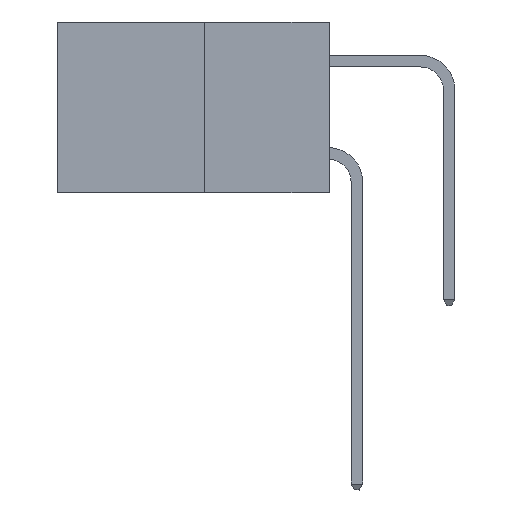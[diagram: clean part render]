
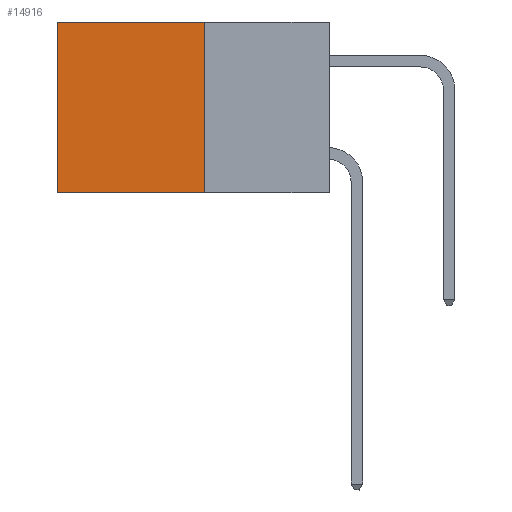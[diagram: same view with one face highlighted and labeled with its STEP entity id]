
A CAD part, left-side view. The second image highlights one B-rep face of the part: STEP entity #14916.
In plain terms, the highlighted planar face has unit normal (-1, 0, 0).
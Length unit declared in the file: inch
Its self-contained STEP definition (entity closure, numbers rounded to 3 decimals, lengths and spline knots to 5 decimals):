
#138 = EDGE_CURVE ( 'NONE', #4573, #4980, #4370, .T. ) ;
#1723 = EDGE_LOOP ( 'NONE', ( #2293, #3855, #4674, #15169 ) ) ;
#1887 = VECTOR ( 'NONE', #6535, 39.37008 ) ;
#2293 = ORIENTED_EDGE ( 'NONE', *, *, #6640, .T. ) ;
#2688 = PLANE ( 'NONE',  #4032 ) ;
#2776 = CARTESIAN_POINT ( 'NONE',  ( 0.277, 0.59, -0.37 ) ) ;
#3490 = EDGE_CURVE ( 'NONE', #12372, #6653, #14640, .T. ) ;
#3855 = ORIENTED_EDGE ( 'NONE', *, *, #138, .F. ) ;
#3945 = DIRECTION ( 'NONE',  ( 1., 0., 0. ) ) ;
#4032 = AXIS2_PLACEMENT_3D ( 'NONE', #12279, #3945, #12329 ) ;
#4370 = LINE ( 'NONE', #10048, #10388 ) ;
#4573 = VERTEX_POINT ( 'NONE', #15115 ) ;
#4631 = LINE ( 'NONE', #2776, #10270 ) ;
#4674 = ORIENTED_EDGE ( 'NONE', *, *, #13037, .F. ) ;
#4980 = VERTEX_POINT ( 'NONE', #5655 ) ;
#5488 = FACE_OUTER_BOUND ( 'NONE', #1723, .T. ) ;
#5655 = CARTESIAN_POINT ( 'NONE',  ( 0.277, 0.59, -0.37 ) ) ;
#6327 = CARTESIAN_POINT ( 'NONE',  ( 0.277, 0.27, -0.37 ) ) ;
#6497 = CARTESIAN_POINT ( 'NONE',  ( 0.277, 0.27, 0. ) ) ;
#6535 = DIRECTION ( 'NONE',  ( 0., 1., 0. ) ) ;
#6640 = EDGE_CURVE ( 'NONE', #6653, #4980, #4631, .T. ) ;
#6653 = VERTEX_POINT ( 'NONE', #13522 ) ;
#7059 = DIRECTION ( 'NONE',  ( 0., 1., 0. ) ) ;
#7214 = VECTOR ( 'NONE', #12225, 39.37008 ) ;
#7593 = LINE ( 'NONE', #6327, #7214 ) ;
#8852 = DIRECTION ( 'NONE',  ( 0., 0., -1. ) ) ;
#10048 = CARTESIAN_POINT ( 'NONE',  ( 0.277, 0.27, -0.37 ) ) ;
#10270 = VECTOR ( 'NONE', #8852, 39.37008 ) ;
#10388 = VECTOR ( 'NONE', #7059, 39.37008 ) ;
#12225 = DIRECTION ( 'NONE',  ( 0., 0., -1. ) ) ;
#12279 = CARTESIAN_POINT ( 'NONE',  ( 0.277, 0.27, -0.37 ) ) ;
#12329 = DIRECTION ( 'NONE',  ( 0., 0., -1. ) ) ;
#12372 = VERTEX_POINT ( 'NONE', #14507 ) ;
#13037 = EDGE_CURVE ( 'NONE', #12372, #4573, #7593, .T. ) ;
#13522 = CARTESIAN_POINT ( 'NONE',  ( 0.277, 0.59, 0. ) ) ;
#14507 = CARTESIAN_POINT ( 'NONE',  ( 0.277, 0.27, 0. ) ) ;
#14640 = LINE ( 'NONE', #6497, #1887 ) ;
#14916 = ADVANCED_FACE ( 'NONE', ( #5488 ), #2688, .F. ) ;
#15115 = CARTESIAN_POINT ( 'NONE',  ( 0.277, 0.27, -0.37 ) ) ;
#15169 = ORIENTED_EDGE ( 'NONE', *, *, #3490, .T. ) ;
